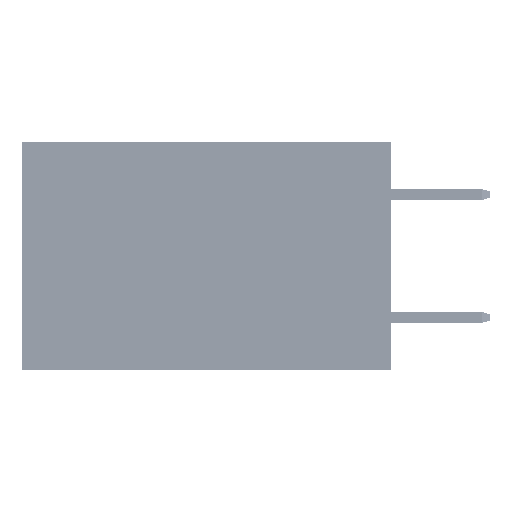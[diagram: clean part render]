
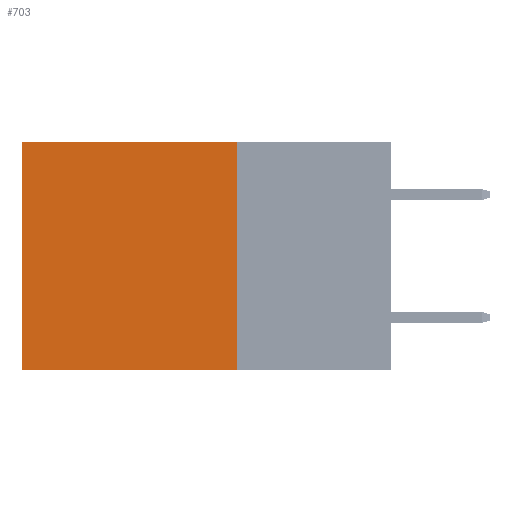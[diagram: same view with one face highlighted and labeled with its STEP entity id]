
A CAD part, left-side view. The second image highlights one B-rep face of the part: STEP entity #703.
In plain terms, the highlighted planar face has unit normal (-1, 0, 0).
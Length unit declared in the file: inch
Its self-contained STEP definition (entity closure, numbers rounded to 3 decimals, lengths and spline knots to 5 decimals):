
#260 = EDGE_CURVE ( 'NONE', #35317, #4722, #39886, .T. ) ;
#703 = ADVANCED_FACE ( 'NONE', ( #35610 ), #12251, .F. ) ;
#1246 = ORIENTED_EDGE ( 'NONE', *, *, #33313, .T. ) ;
#2520 = CARTESIAN_POINT ( 'NONE',  ( 0.2875, 0.25, 0. ) ) ;
#3191 = DIRECTION ( 'NONE',  ( 0., 1., 0. ) ) ;
#3888 = CARTESIAN_POINT ( 'NONE',  ( 0.2875, 0.25, -0.37 ) ) ;
#3910 = CARTESIAN_POINT ( 'NONE',  ( 0.2875, 0.6, 0. ) ) ;
#4474 = CARTESIAN_POINT ( 'NONE',  ( 0.2875, 0.25, 0. ) ) ;
#4722 = VERTEX_POINT ( 'NONE', #10435 ) ;
#5914 = VECTOR ( 'NONE', #43496, 39.37008 ) ;
#7224 = CARTESIAN_POINT ( 'NONE',  ( 0.2875, 0.6, 0. ) ) ;
#8015 = EDGE_CURVE ( 'NONE', #4722, #22975, #12700, .T. ) ;
#8956 = CARTESIAN_POINT ( 'NONE',  ( 0.2875, 0.25, 0. ) ) ;
#10435 = CARTESIAN_POINT ( 'NONE',  ( 0.2875, 0.25, -0.37 ) ) ;
#10436 = ORIENTED_EDGE ( 'NONE', *, *, #8015, .F. ) ;
#12251 = PLANE ( 'NONE',  #46255 ) ;
#12420 = DIRECTION ( 'NONE',  ( 1., 0., 0. ) ) ;
#12700 = LINE ( 'NONE', #3888, #5914 ) ;
#15475 = VERTEX_POINT ( 'NONE', #3910 ) ;
#16758 = ORIENTED_EDGE ( 'NONE', *, *, #260, .F. ) ;
#20604 = LINE ( 'NONE', #7224, #36703 ) ;
#21860 = VECTOR ( 'NONE', #3191, 39.37008 ) ;
#22201 = CARTESIAN_POINT ( 'NONE',  ( 0.2875, 0.6, -0.37 ) ) ;
#22975 = VERTEX_POINT ( 'NONE', #22201 ) ;
#23824 = DIRECTION ( 'NONE',  ( 0., 0., -1. ) ) ;
#24262 = EDGE_CURVE ( 'NONE', #35317, #15475, #48526, .T. ) ;
#26806 = VECTOR ( 'NONE', #36965, 39.37008 ) ;
#33313 = EDGE_CURVE ( 'NONE', #15475, #22975, #20604, .T. ) ;
#35308 = EDGE_LOOP ( 'NONE', ( #1246, #10436, #16758, #50789 ) ) ;
#35317 = VERTEX_POINT ( 'NONE', #4474 ) ;
#35610 = FACE_OUTER_BOUND ( 'NONE', #35308, .T. ) ;
#36703 = VECTOR ( 'NONE', #39214, 39.37008 ) ;
#36965 = DIRECTION ( 'NONE',  ( 0., 0., -1. ) ) ;
#39214 = DIRECTION ( 'NONE',  ( 0., 0., -1. ) ) ;
#39886 = LINE ( 'NONE', #8956, #26806 ) ;
#43496 = DIRECTION ( 'NONE',  ( 0., 1., 0. ) ) ;
#44260 = CARTESIAN_POINT ( 'NONE',  ( 0.2875, 0.25, 0. ) ) ;
#46255 = AXIS2_PLACEMENT_3D ( 'NONE', #44260, #12420, #23824 ) ;
#48526 = LINE ( 'NONE', #2520, #21860 ) ;
#50789 = ORIENTED_EDGE ( 'NONE', *, *, #24262, .T. ) ;
